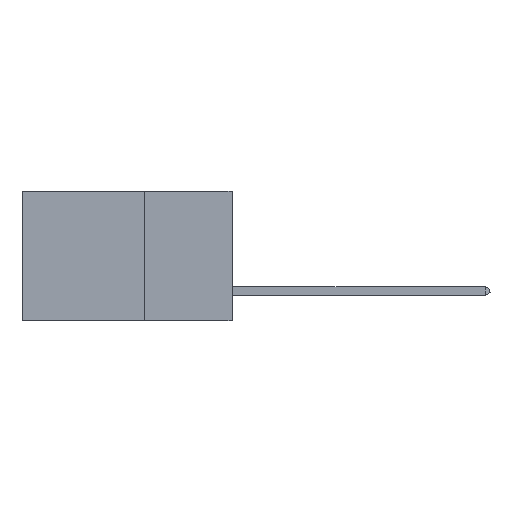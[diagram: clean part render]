
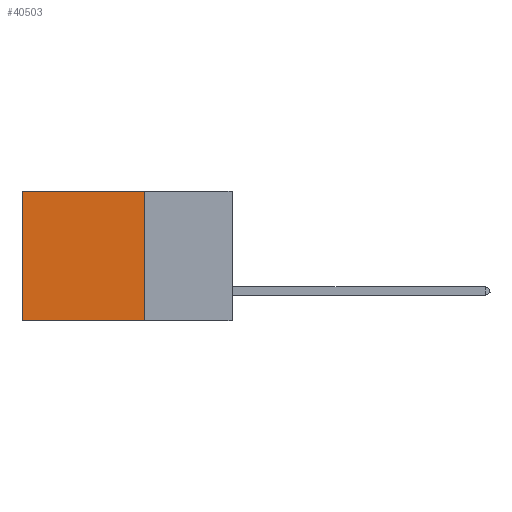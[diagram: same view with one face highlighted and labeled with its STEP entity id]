
A CAD part, left-side view. The second image highlights one B-rep face of the part: STEP entity #40503.
In plain terms, the highlighted planar face has unit normal (-1, 0, 0).
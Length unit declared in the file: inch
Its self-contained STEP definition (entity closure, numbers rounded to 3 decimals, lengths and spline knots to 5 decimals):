
#137 = EDGE_CURVE ( 'NONE', #14225, #38258, #7156, .T. ) ;
#392 = CARTESIAN_POINT ( 'NONE',  ( 0.2875, 0.25, 0. ) ) ;
#648 = LINE ( 'NONE', #15311, #39254 ) ;
#4780 = CARTESIAN_POINT ( 'NONE',  ( 0.2875, 0.6, -0.37 ) ) ;
#6404 = VECTOR ( 'NONE', #27750, 39.37008 ) ;
#7156 = LINE ( 'NONE', #7164, #48138 ) ;
#7164 = CARTESIAN_POINT ( 'NONE',  ( 0.2875, 0.25, -0.37 ) ) ;
#8428 = CARTESIAN_POINT ( 'NONE',  ( 0.2875, 0.25, 0. ) ) ;
#9989 = LINE ( 'NONE', #8428, #6404 ) ;
#10892 = CARTESIAN_POINT ( 'NONE',  ( 0.2875, 0.25, -0.37 ) ) ;
#14225 = VERTEX_POINT ( 'NONE', #10892 ) ;
#15311 = CARTESIAN_POINT ( 'NONE',  ( 0.2875, 0.6, 0. ) ) ;
#17318 = ORIENTED_EDGE ( 'NONE', *, *, #46462, .F. ) ;
#19041 = LINE ( 'NONE', #36729, #37142 ) ;
#19695 = DIRECTION ( 'NONE',  ( 0., 0., -1. ) ) ;
#20174 = CARTESIAN_POINT ( 'NONE',  ( 0.2875, 0.6, 0. ) ) ;
#25106 = DIRECTION ( 'NONE',  ( 0., 0., -1. ) ) ;
#25507 = ORIENTED_EDGE ( 'NONE', *, *, #28608, .T. ) ;
#25824 = DIRECTION ( 'NONE',  ( 0., 1., 0. ) ) ;
#27750 = DIRECTION ( 'NONE',  ( 0., 1., 0. ) ) ;
#28608 = EDGE_CURVE ( 'NONE', #30725, #38258, #648, .T. ) ;
#28872 = ORIENTED_EDGE ( 'NONE', *, *, #137, .F. ) ;
#30725 = VERTEX_POINT ( 'NONE', #20174 ) ;
#31191 = FACE_OUTER_BOUND ( 'NONE', #42055, .T. ) ;
#32236 = CARTESIAN_POINT ( 'NONE',  ( 0.2875, 0.25, 0. ) ) ;
#35034 = EDGE_CURVE ( 'NONE', #39842, #30725, #9989, .T. ) ;
#35325 = ORIENTED_EDGE ( 'NONE', *, *, #35034, .T. ) ;
#36729 = CARTESIAN_POINT ( 'NONE',  ( 0.2875, 0.25, 0. ) ) ;
#37142 = VECTOR ( 'NONE', #25106, 39.37008 ) ;
#38258 = VERTEX_POINT ( 'NONE', #4780 ) ;
#39236 = AXIS2_PLACEMENT_3D ( 'NONE', #32236, #47457, #43892 ) ;
#39254 = VECTOR ( 'NONE', #19695, 39.37008 ) ;
#39842 = VERTEX_POINT ( 'NONE', #392 ) ;
#40025 = PLANE ( 'NONE',  #39236 ) ;
#40503 = ADVANCED_FACE ( 'NONE', ( #31191 ), #40025, .F. ) ;
#42055 = EDGE_LOOP ( 'NONE', ( #25507, #28872, #17318, #35325 ) ) ;
#43892 = DIRECTION ( 'NONE',  ( 0., 0., -1. ) ) ;
#46462 = EDGE_CURVE ( 'NONE', #39842, #14225, #19041, .T. ) ;
#47457 = DIRECTION ( 'NONE',  ( 1., 0., 0. ) ) ;
#48138 = VECTOR ( 'NONE', #25824, 39.37008 ) ;
